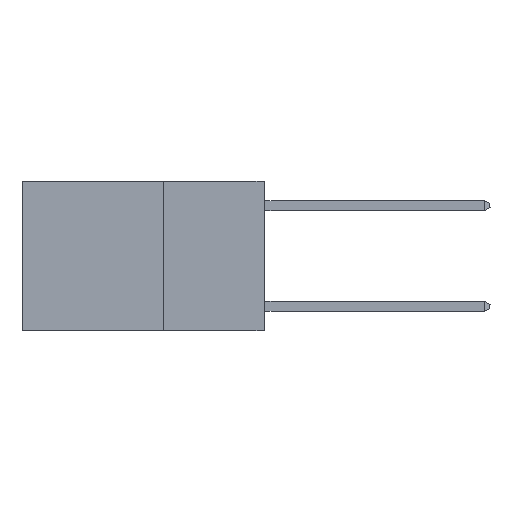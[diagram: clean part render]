
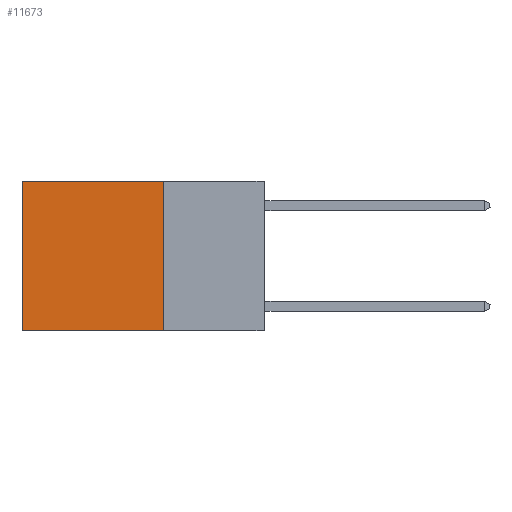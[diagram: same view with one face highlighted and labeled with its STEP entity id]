
A CAD part, left-side view. The second image highlights one B-rep face of the part: STEP entity #11673.
In plain terms, the highlighted planar face has unit normal (-1, 0, 0).
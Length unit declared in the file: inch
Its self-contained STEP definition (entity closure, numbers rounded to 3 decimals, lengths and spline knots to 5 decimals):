
#286 = EDGE_CURVE ( 'NONE', #26062, #6837, #23134, .T. ) ;
#1074 = FACE_OUTER_BOUND ( 'NONE', #13497, .T. ) ;
#1359 = CARTESIAN_POINT ( 'NONE',  ( 0.2625, 0.25, 0. ) ) ;
#1373 = VERTEX_POINT ( 'NONE', #15116 ) ;
#1523 = LINE ( 'NONE', #15191, #5137 ) ;
#1873 = EDGE_CURVE ( 'NONE', #5063, #1373, #26450, .T. ) ;
#1917 = ORIENTED_EDGE ( 'NONE', *, *, #1873, .T. ) ;
#3455 = DIRECTION ( 'NONE',  ( 0., 0., -1. ) ) ;
#3944 = DIRECTION ( 'NONE',  ( 0., 1., 0. ) ) ;
#5063 = VERTEX_POINT ( 'NONE', #14893 ) ;
#5137 = VECTOR ( 'NONE', #10873, 39.37008 ) ;
#6837 = VERTEX_POINT ( 'NONE', #14136 ) ;
#7261 = VECTOR ( 'NONE', #18287, 39.37008 ) ;
#7885 = VECTOR ( 'NONE', #11676, 39.37008 ) ;
#8048 = PLANE ( 'NONE',  #27889 ) ;
#9522 = LINE ( 'NONE', #25164, #7261 ) ;
#9712 = ORIENTED_EDGE ( 'NONE', *, *, #27274, .F. ) ;
#10327 = CARTESIAN_POINT ( 'NONE',  ( 0.2625, 0.25, 0. ) ) ;
#10873 = DIRECTION ( 'NONE',  ( 0., 0., -1. ) ) ;
#11673 = ADVANCED_FACE ( 'NONE', ( #1074 ), #8048, .F. ) ;
#11676 = DIRECTION ( 'NONE',  ( 0., 1., 0. ) ) ;
#13497 = EDGE_LOOP ( 'NONE', ( #26550, #17106, #9712, #1917 ) ) ;
#14082 = CARTESIAN_POINT ( 'NONE',  ( 0.2625, 0.25, -0.37 ) ) ;
#14136 = CARTESIAN_POINT ( 'NONE',  ( 0.2625, 0.6, -0.37 ) ) ;
#14893 = CARTESIAN_POINT ( 'NONE',  ( 0.2625, 0.25, 0. ) ) ;
#15116 = CARTESIAN_POINT ( 'NONE',  ( 0.2625, 0.6, 0. ) ) ;
#15191 = CARTESIAN_POINT ( 'NONE',  ( 0.2625, 0.25, 0. ) ) ;
#17106 = ORIENTED_EDGE ( 'NONE', *, *, #286, .F. ) ;
#17942 = VECTOR ( 'NONE', #3944, 39.37008 ) ;
#18287 = DIRECTION ( 'NONE',  ( 0., 0., -1. ) ) ;
#21293 = EDGE_CURVE ( 'NONE', #1373, #6837, #9522, .T. ) ;
#23134 = LINE ( 'NONE', #25970, #7885 ) ;
#25164 = CARTESIAN_POINT ( 'NONE',  ( 0.2625, 0.6, 0. ) ) ;
#25807 = DIRECTION ( 'NONE',  ( 1., 0., 0. ) ) ;
#25970 = CARTESIAN_POINT ( 'NONE',  ( 0.2625, 0.25, -0.37 ) ) ;
#26062 = VERTEX_POINT ( 'NONE', #14082 ) ;
#26450 = LINE ( 'NONE', #10327, #17942 ) ;
#26550 = ORIENTED_EDGE ( 'NONE', *, *, #21293, .T. ) ;
#27274 = EDGE_CURVE ( 'NONE', #5063, #26062, #1523, .T. ) ;
#27889 = AXIS2_PLACEMENT_3D ( 'NONE', #1359, #25807, #3455 ) ;
